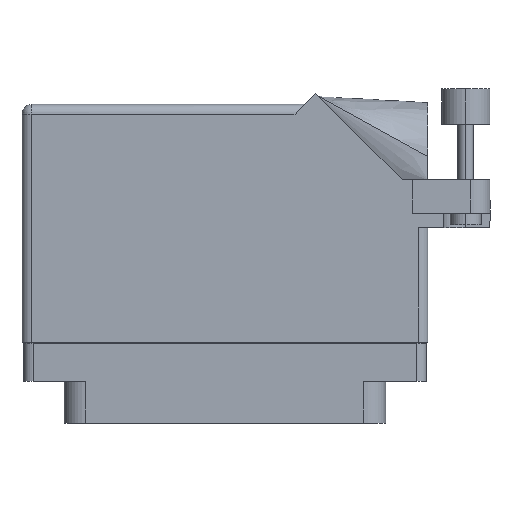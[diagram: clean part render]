
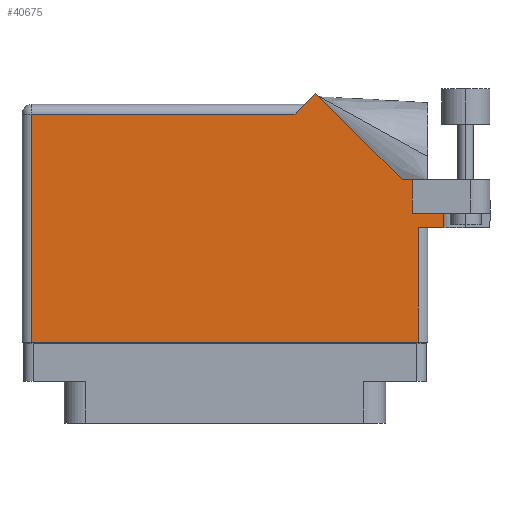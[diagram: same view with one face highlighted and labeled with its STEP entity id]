
A CAD part, front view. The second image highlights one B-rep face of the part: STEP entity #40675.
In plain terms, the highlighted face is planar.
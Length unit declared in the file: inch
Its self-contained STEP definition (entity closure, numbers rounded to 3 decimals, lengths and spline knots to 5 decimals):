
#621 = ORIENTED_EDGE ( 'NONE', *, *, #31453, .T. ) ;
#1182 = CARTESIAN_POINT ( 'NONE',  ( 1.206, 0.731, 0.455 ) ) ;
#1700 = ORIENTED_EDGE ( 'NONE', *, *, #28150, .F. ) ;
#1770 = CARTESIAN_POINT ( 'NONE',  ( 1.206, 0.944, 0.455 ) ) ;
#2472 = CARTESIAN_POINT ( 'NONE',  ( 1.206, 0.731, 0.455 ) ) ;
#2956 = EDGE_CURVE ( 'NONE', #18296, #5849, #28794, .T. ) ;
#3626 = VERTEX_POINT ( 'NONE', #30800 ) ;
#4063 = CARTESIAN_POINT ( 'NONE',  ( -1.244, 1.368, 0.455 ) ) ;
#4371 = LINE ( 'NONE', #34602, #24943 ) ;
#4567 = FACE_OUTER_BOUND ( 'NONE', #40174, .T. ) ;
#4752 = PLANE ( 'NONE',  #15110 ) ;
#5763 = ORIENTED_EDGE ( 'NONE', *, *, #2956, .T. ) ;
#5849 = VERTEX_POINT ( 'NONE', #19412 ) ;
#6048 = ORIENTED_EDGE ( 'NONE', *, *, #30330, .F. ) ;
#7085 = VECTOR ( 'NONE', #24781, 39.37008 ) ;
#7428 = CARTESIAN_POINT ( 'NONE',  ( 1.14042, 0.944, 0.455 ) ) ;
#7670 = LINE ( 'NONE', #2472, #35705 ) ;
#8028 = CARTESIAN_POINT ( 'NONE',  ( 1.244, -0.1, 0.455 ) ) ;
#8376 = ORIENTED_EDGE ( 'NONE', *, *, #38971, .T. ) ;
#8893 = VERTEX_POINT ( 'NONE', #42294 ) ;
#9228 = DIRECTION ( 'NONE',  ( -0.707, -0.707, 0. ) ) ;
#11982 = DIRECTION ( 'NONE',  ( 1., 0., 0. ) ) ;
#13027 = VECTOR ( 'NONE', #39516, 39.37008 ) ;
#13286 = VERTEX_POINT ( 'NONE', #1182 ) ;
#15049 = LINE ( 'NONE', #26250, #35716 ) ;
#15110 = AXIS2_PLACEMENT_3D ( 'NONE', #32189, #35168, #38584 ) ;
#15586 = DIRECTION ( 'NONE',  ( 1., 0., 0. ) ) ;
#15682 = CARTESIAN_POINT ( 'NONE',  ( 1.244, 0.637, 0.455 ) ) ;
#16115 = CARTESIAN_POINT ( 'NONE',  ( 1.4075, 1.06177, 0.455 ) ) ;
#16260 = VERTEX_POINT ( 'NONE', #39958 ) ;
#18296 = VERTEX_POINT ( 'NONE', #21226 ) ;
#19011 = LINE ( 'NONE', #30860, #42813 ) ;
#19143 = VECTOR ( 'NONE', #11982, 39.37008 ) ;
#19412 = CARTESIAN_POINT ( 'NONE',  ( 0.58371, 1.50071, 0.455 ) ) ;
#20254 = VECTOR ( 'NONE', #22342, 39.37008 ) ;
#20312 = ORIENTED_EDGE ( 'NONE', *, *, #24289, .T. ) ;
#21059 = CARTESIAN_POINT ( 'NONE',  ( -1.306, -0.1, 0.455 ) ) ;
#21149 = VERTEX_POINT ( 'NONE', #1770 ) ;
#21226 = CARTESIAN_POINT ( 'NONE',  ( 1.14042, 0.944, 0.455 ) ) ;
#21277 = DIRECTION ( 'NONE',  ( 0., 1., 0. ) ) ;
#21636 = LINE ( 'NONE', #32096, #36504 ) ;
#21749 = LINE ( 'NONE', #38887, #19143 ) ;
#22342 = DIRECTION ( 'NONE',  ( 0., -1., 0. ) ) ;
#23081 = VECTOR ( 'NONE', #15586, 39.37008 ) ;
#24114 = LINE ( 'NONE', #15682, #13027 ) ;
#24289 = EDGE_CURVE ( 'NONE', #13286, #21149, #4371, .T. ) ;
#24473 = VERTEX_POINT ( 'NONE', #38892 ) ;
#24781 = DIRECTION ( 'NONE',  ( 0., -1., 0. ) ) ;
#24943 = VECTOR ( 'NONE', #21277, 39.37008 ) ;
#25050 = LINE ( 'NONE', #35306, #7085 ) ;
#26250 = CARTESIAN_POINT ( 'NONE',  ( 0.513, 1.43, 0.455 ) ) ;
#26517 = DIRECTION ( 'NONE',  ( 1., 0., 0. ) ) ;
#27149 = ORIENTED_EDGE ( 'NONE', *, *, #32615, .T. ) ;
#27714 = EDGE_CURVE ( 'NONE', #38282, #24473, #24114, .T. ) ;
#28150 = EDGE_CURVE ( 'NONE', #13286, #16260, #7670, .T. ) ;
#28794 = LINE ( 'NONE', #7428, #42531 ) ;
#30330 = EDGE_CURVE ( 'NONE', #16260, #3626, #39303, .T. ) ;
#30800 = CARTESIAN_POINT ( 'NONE',  ( 1.4075, 0.637, 0.455 ) ) ;
#30860 = CARTESIAN_POINT ( 'NONE',  ( -1.306, 1.368, 0.455 ) ) ;
#31020 = DIRECTION ( 'NONE',  ( -0.707, 0.707, 0. ) ) ;
#31453 = EDGE_CURVE ( 'NONE', #24473, #3626, #21749, .T. ) ;
#32096 = CARTESIAN_POINT ( 'NONE',  ( 1.706, 0.944, 0.455 ) ) ;
#32189 = CARTESIAN_POINT ( 'NONE',  ( -1.306, 1.43, 0.455 ) ) ;
#32609 = LINE ( 'NONE', #21059, #23081 ) ;
#32615 = EDGE_CURVE ( 'NONE', #21149, #18296, #21636, .T. ) ;
#33541 = ORIENTED_EDGE ( 'NONE', *, *, #39803, .T. ) ;
#33712 = VERTEX_POINT ( 'NONE', #4063 ) ;
#34034 = EDGE_CURVE ( 'NONE', #8893, #38282, #32609, .T. ) ;
#34602 = CARTESIAN_POINT ( 'NONE',  ( 1.206, 0.731, 0.455 ) ) ;
#35168 = DIRECTION ( 'NONE',  ( 0., 0., -1. ) ) ;
#35306 = CARTESIAN_POINT ( 'NONE',  ( -1.244, -0.1, 0.455 ) ) ;
#35327 = DIRECTION ( 'NONE',  ( -1., 0., 0. ) ) ;
#35705 = VECTOR ( 'NONE', #26517, 39.37008 ) ;
#35716 = VECTOR ( 'NONE', #9228, 39.37008 ) ;
#35995 = VERTEX_POINT ( 'NONE', #41106 ) ;
#36504 = VECTOR ( 'NONE', #42752, 39.37008 ) ;
#38072 = ORIENTED_EDGE ( 'NONE', *, *, #34034, .T. ) ;
#38282 = VERTEX_POINT ( 'NONE', #8028 ) ;
#38584 = DIRECTION ( 'NONE',  ( -1., 0., 0. ) ) ;
#38887 = CARTESIAN_POINT ( 'NONE',  ( 1.306, 0.637, 0.455 ) ) ;
#38892 = CARTESIAN_POINT ( 'NONE',  ( 1.244, 0.637, 0.455 ) ) ;
#38971 = EDGE_CURVE ( 'NONE', #5849, #35995, #15049, .T. ) ;
#39303 = LINE ( 'NONE', #16115, #20254 ) ;
#39516 = DIRECTION ( 'NONE',  ( 0., 1., 0. ) ) ;
#39803 = EDGE_CURVE ( 'NONE', #33712, #8893, #25050, .T. ) ;
#39958 = CARTESIAN_POINT ( 'NONE',  ( 1.4075, 0.731, 0.455 ) ) ;
#40174 = EDGE_LOOP ( 'NONE', ( #38072, #41887, #621, #6048, #1700, #20312, #27149, #5763, #8376, #41866, #33541 ) ) ;
#40675 = ADVANCED_FACE ( 'NONE', ( #4567 ), #4752, .F. ) ;
#41106 = CARTESIAN_POINT ( 'NONE',  ( 0.451, 1.368, 0.455 ) ) ;
#41866 = ORIENTED_EDGE ( 'NONE', *, *, #43568, .T. ) ;
#41887 = ORIENTED_EDGE ( 'NONE', *, *, #27714, .T. ) ;
#42294 = CARTESIAN_POINT ( 'NONE',  ( -1.244, -0.1, 0.455 ) ) ;
#42531 = VECTOR ( 'NONE', #31020, 39.37008 ) ;
#42752 = DIRECTION ( 'NONE',  ( -1., 0., 0. ) ) ;
#42813 = VECTOR ( 'NONE', #35327, 39.37008 ) ;
#43568 = EDGE_CURVE ( 'NONE', #35995, #33712, #19011, .T. ) ;
